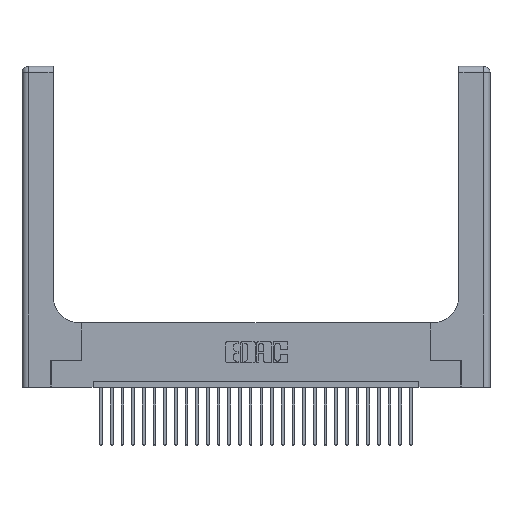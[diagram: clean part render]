
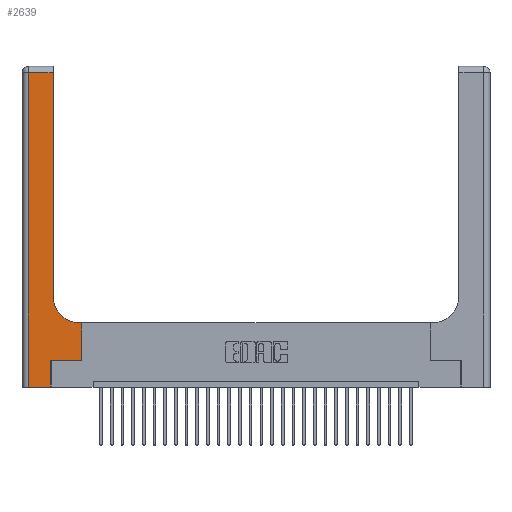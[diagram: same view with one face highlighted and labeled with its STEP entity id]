
A CAD part, top view. The second image highlights one B-rep face of the part: STEP entity #2639.
In plain terms, the highlighted planar face has unit normal (0, 0, 1).
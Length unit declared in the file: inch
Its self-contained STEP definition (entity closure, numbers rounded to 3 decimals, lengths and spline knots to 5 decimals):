
#19 = CIRCLE ( 'NONE', #6697, 0.25 ) ;
#117 = VERTEX_POINT ( 'NONE', #13095 ) ;
#1153 = ORIENTED_EDGE ( 'NONE', *, *, #9433, .T. ) ;
#1365 = DIRECTION ( 'NONE',  ( 0., 1., 0. ) ) ;
#1491 = DIRECTION ( 'NONE',  ( 1., 0., 0. ) ) ;
#1503 = ORIENTED_EDGE ( 'NONE', *, *, #2674, .T. ) ;
#2123 = CARTESIAN_POINT ( 'NONE',  ( 0.5585, 0.6, 0.37 ) ) ;
#2175 = DIRECTION ( 'NONE',  ( -1., 0., 0. ) ) ;
#2429 = CARTESIAN_POINT ( 'NONE',  ( 0.06, 3., 0.37 ) ) ;
#2537 = DIRECTION ( 'NONE',  ( -1., 0., 0. ) ) ;
#2639 = ADVANCED_FACE ( 'NONE', ( #8909 ), #19225, .F. ) ;
#2674 = EDGE_CURVE ( 'NONE', #20719, #19749, #9281, .T. ) ;
#2983 = DIRECTION ( 'NONE',  ( 1., 0., 0. ) ) ;
#3216 = ORIENTED_EDGE ( 'NONE', *, *, #6543, .T. ) ;
#3312 = CARTESIAN_POINT ( 'NONE',  ( 0.2915, 2.94, 0.37 ) ) ;
#3424 = DIRECTION ( 'NONE',  ( -1., 0., 0. ) ) ;
#4286 = DIRECTION ( 'NONE',  ( 0., 1., 0. ) ) ;
#4441 = EDGE_CURVE ( 'NONE', #6948, #21985, #13086, .T. ) ;
#5729 = CARTESIAN_POINT ( 'NONE',  ( 0., 3., 0.37 ) ) ;
#5784 = CARTESIAN_POINT ( 'NONE',  ( 0.2915, 0.85, 0.37 ) ) ;
#6543 = EDGE_CURVE ( 'NONE', #117, #19660, #12670, .T. ) ;
#6697 = AXIS2_PLACEMENT_3D ( 'NONE', #18916, #14450, #22089 ) ;
#6948 = VERTEX_POINT ( 'NONE', #5784 ) ;
#6987 = CARTESIAN_POINT ( 'NONE',  ( 0.2915, 0.6, 0.37 ) ) ;
#7208 = DIRECTION ( 'NONE',  ( 0., -1., 0. ) ) ;
#8187 = EDGE_CURVE ( 'NONE', #19660, #17931, #15779, .T. ) ;
#8472 = ORIENTED_EDGE ( 'NONE', *, *, #4441, .T. ) ;
#8785 = ORIENTED_EDGE ( 'NONE', *, *, #26719, .T. ) ;
#8876 = VECTOR ( 'NONE', #2537, 39.37008 ) ;
#8909 = FACE_OUTER_BOUND ( 'NONE', #24926, .T. ) ;
#9119 = ORIENTED_EDGE ( 'NONE', *, *, #8187, .T. ) ;
#9281 = LINE ( 'NONE', #12128, #18517 ) ;
#9433 = EDGE_CURVE ( 'NONE', #16525, #6948, #19, .T. ) ;
#10191 = DIRECTION ( 'NONE',  ( 0., 0., -1. ) ) ;
#10620 = VECTOR ( 'NONE', #4286, 39.37008 ) ;
#10701 = CARTESIAN_POINT ( 'NONE',  ( 0.269, 0., 0.37 ) ) ;
#11264 = DIRECTION ( 'NONE',  ( 0., 1., 0. ) ) ;
#11337 = CARTESIAN_POINT ( 'NONE',  ( 0.269, 0., 0.37 ) ) ;
#11368 = ORIENTED_EDGE ( 'NONE', *, *, #27710, .T. ) ;
#11606 = VECTOR ( 'NONE', #1491, 39.37008 ) ;
#12128 = CARTESIAN_POINT ( 'NONE',  ( 0., 0., 0.37 ) ) ;
#12314 = ORIENTED_EDGE ( 'NONE', *, *, #12343, .T. ) ;
#12343 = EDGE_CURVE ( 'NONE', #17931, #16525, #21331, .T. ) ;
#12592 = CARTESIAN_POINT ( 'NONE',  ( 0.5585, 0.25, 0.37 ) ) ;
#12670 = LINE ( 'NONE', #12818, #11606 ) ;
#12818 = CARTESIAN_POINT ( 'NONE',  ( 0.269, 0.25, 0.37 ) ) ;
#12843 = VECTOR ( 'NONE', #2175, 39.37008 ) ;
#13086 = LINE ( 'NONE', #27031, #10620 ) ;
#13095 = CARTESIAN_POINT ( 'NONE',  ( 0.269, 0.25, 0.37 ) ) ;
#13432 = CARTESIAN_POINT ( 'NONE',  ( 0.06, 2.94, 0.37 ) ) ;
#14450 = DIRECTION ( 'NONE',  ( 0., 0., -1. ) ) ;
#15779 = LINE ( 'NONE', #12592, #22858 ) ;
#16525 = VERTEX_POINT ( 'NONE', #26144 ) ;
#17931 = VERTEX_POINT ( 'NONE', #2123 ) ;
#18517 = VECTOR ( 'NONE', #2983, 39.37008 ) ;
#18744 = CARTESIAN_POINT ( 'NONE',  ( 0.06, 0., 0.37 ) ) ;
#18867 = VECTOR ( 'NONE', #11264, 39.37008 ) ;
#18888 = LINE ( 'NONE', #25050, #12843 ) ;
#18916 = CARTESIAN_POINT ( 'NONE',  ( 0.5415, 0.85, 0.37 ) ) ;
#19225 = PLANE ( 'NONE',  #28262 ) ;
#19660 = VERTEX_POINT ( 'NONE', #21989 ) ;
#19749 = VERTEX_POINT ( 'NONE', #11337 ) ;
#20719 = VERTEX_POINT ( 'NONE', #18744 ) ;
#21331 = LINE ( 'NONE', #6987, #8876 ) ;
#21985 = VERTEX_POINT ( 'NONE', #3312 ) ;
#21989 = CARTESIAN_POINT ( 'NONE',  ( 0.5585, 0.25, 0.37 ) ) ;
#22089 = DIRECTION ( 'NONE',  ( 1., 0., 0. ) ) ;
#22097 = VECTOR ( 'NONE', #7208, 39.37008 ) ;
#22136 = VERTEX_POINT ( 'NONE', #13432 ) ;
#22858 = VECTOR ( 'NONE', #1365, 39.37008 ) ;
#24344 = ORIENTED_EDGE ( 'NONE', *, *, #27320, .T. ) ;
#24926 = EDGE_LOOP ( 'NONE', ( #8472, #8785, #24344, #1503, #11368, #3216, #9119, #12314, #1153 ) ) ;
#25050 = CARTESIAN_POINT ( 'NONE',  ( 0., 2.94, 0.37 ) ) ;
#26144 = CARTESIAN_POINT ( 'NONE',  ( 0.5415, 0.6, 0.37 ) ) ;
#26385 = LINE ( 'NONE', #2429, #22097 ) ;
#26719 = EDGE_CURVE ( 'NONE', #21985, #22136, #18888, .T. ) ;
#27031 = CARTESIAN_POINT ( 'NONE',  ( 0.2915, 3., 0.37 ) ) ;
#27320 = EDGE_CURVE ( 'NONE', #22136, #20719, #26385, .T. ) ;
#27710 = EDGE_CURVE ( 'NONE', #19749, #117, #27726, .T. ) ;
#27726 = LINE ( 'NONE', #10701, #18867 ) ;
#28262 = AXIS2_PLACEMENT_3D ( 'NONE', #5729, #10191, #3424 ) ;
